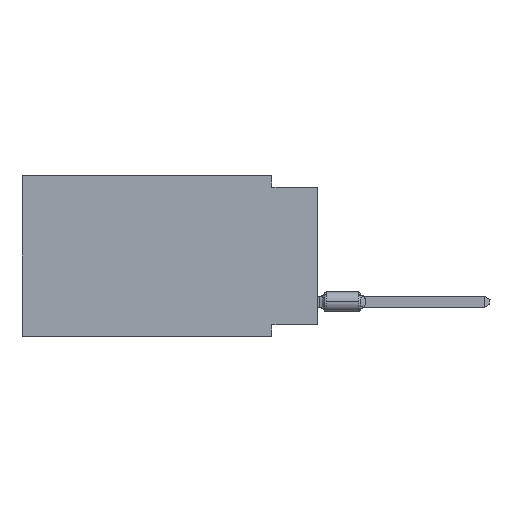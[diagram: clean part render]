
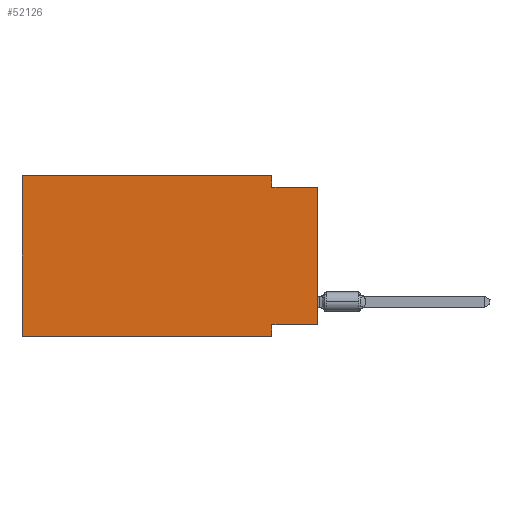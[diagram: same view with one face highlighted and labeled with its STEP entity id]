
A CAD part, left-side view. The second image highlights one B-rep face of the part: STEP entity #52126.
In plain terms, the highlighted planar face has unit normal (-1, 0, 0).
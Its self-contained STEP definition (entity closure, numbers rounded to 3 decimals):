
#1 = VECTOR ( 'NONE', #99394, 1000. ) ;
#1912 = VERTEX_POINT ( 'NONE', #21549 ) ;
#3960 = ORIENTED_EDGE ( 'NONE', *, *, #40717, .F. ) ;
#4182 = DIRECTION ( 'NONE',  ( 0., 0., -1. ) ) ;
#7124 = VERTEX_POINT ( 'NONE', #81972 ) ;
#7628 = ORIENTED_EDGE ( 'NONE', *, *, #89636, .F. ) ;
#10782 = DIRECTION ( 'NONE',  ( 0., 0., -1. ) ) ;
#10893 = LINE ( 'NONE', #11415, #1 ) ;
#11415 = CARTESIAN_POINT ( 'NONE',  ( 0., 0., -0.635 ) ) ;
#11553 = CARTESIAN_POINT ( 'NONE',  ( 0., 16.383, 0. ) ) ;
#11763 = CARTESIAN_POINT ( 'NONE',  ( 0., 16.383, 0. ) ) ;
#11833 = LINE ( 'NONE', #36059, #82247 ) ;
#12794 = VERTEX_POINT ( 'NONE', #13997 ) ;
#13997 = CARTESIAN_POINT ( 'NONE',  ( 0., 16.383, -8.89 ) ) ;
#14413 = VERTEX_POINT ( 'NONE', #46054 ) ;
#17647 = EDGE_CURVE ( 'NONE', #39506, #90280, #42423, .T. ) ;
#17708 = EDGE_CURVE ( 'NONE', #12794, #90280, #11833, .T. ) ;
#17879 = VECTOR ( 'NONE', #26842, 1000. ) ;
#18206 = ORIENTED_EDGE ( 'NONE', *, *, #17708, .T. ) ;
#19656 = FACE_OUTER_BOUND ( 'NONE', #53741, .T. ) ;
#19682 = CARTESIAN_POINT ( 'NONE',  ( 0., 16.383, 0. ) ) ;
#21549 = CARTESIAN_POINT ( 'NONE',  ( 0., 0., -0.635 ) ) ;
#24743 = VERTEX_POINT ( 'NONE', #36303 ) ;
#26842 = DIRECTION ( 'NONE',  ( 0., 0., 1. ) ) ;
#27424 = EDGE_CURVE ( 'NONE', #7124, #55537, #98212, .T. ) ;
#28751 = ORIENTED_EDGE ( 'NONE', *, *, #27424, .F. ) ;
#29482 = EDGE_CURVE ( 'NONE', #24743, #1912, #68447, .T. ) ;
#36059 = CARTESIAN_POINT ( 'NONE',  ( 0., 16.383, -8.89 ) ) ;
#36303 = CARTESIAN_POINT ( 'NONE',  ( 0., 0., -8.255 ) ) ;
#37333 = DIRECTION ( 'NONE',  ( 0., 0., 1. ) ) ;
#39506 = VERTEX_POINT ( 'NONE', #102109 ) ;
#40717 = EDGE_CURVE ( 'NONE', #12794, #7124, #44740, .T. ) ;
#42423 = LINE ( 'NONE', #82987, #55319 ) ;
#43921 = DIRECTION ( 'NONE',  ( 1., 0., 0. ) ) ;
#44740 = LINE ( 'NONE', #11553, #17879 ) ;
#46054 = CARTESIAN_POINT ( 'NONE',  ( 0., 2.54, -0.635 ) ) ;
#46403 = CARTESIAN_POINT ( 'NONE',  ( 0., 0., -8.255 ) ) ;
#49022 = VECTOR ( 'NONE', #68158, 1000. ) ;
#52126 = ADVANCED_FACE ( 'NONE', ( #19656 ), #83963, .F. ) ;
#52921 = DIRECTION ( 'NONE',  ( 0., -1., 0. ) ) ;
#53741 = EDGE_LOOP ( 'NONE', ( #103125, #98669, #7628, #28751, #3960, #18206, #103099, #67487 ) ) ;
#54201 = CARTESIAN_POINT ( 'NONE',  ( 0., 0., 0. ) ) ;
#54928 = VECTOR ( 'NONE', #4182, 1000. ) ;
#55319 = VECTOR ( 'NONE', #10782, 1000. ) ;
#55537 = VERTEX_POINT ( 'NONE', #89894 ) ;
#60238 = EDGE_CURVE ( 'NONE', #24743, #39506, #62213, .T. ) ;
#62213 = LINE ( 'NONE', #46403, #78360 ) ;
#62346 = AXIS2_PLACEMENT_3D ( 'NONE', #11763, #43921, #76046 ) ;
#65824 = CARTESIAN_POINT ( 'NONE',  ( 0., 2.54, -8.89 ) ) ;
#67487 = ORIENTED_EDGE ( 'NONE', *, *, #60238, .F. ) ;
#68158 = DIRECTION ( 'NONE',  ( 0., -1., 0. ) ) ;
#68447 = LINE ( 'NONE', #54201, #87966 ) ;
#69592 = DIRECTION ( 'NONE',  ( 0., 1., 0. ) ) ;
#72010 = EDGE_CURVE ( 'NONE', #14413, #1912, #10893, .T. ) ;
#76046 = DIRECTION ( 'NONE',  ( 0., 0., -1. ) ) ;
#76363 = CARTESIAN_POINT ( 'NONE',  ( 0., 2.54, 0. ) ) ;
#76884 = LINE ( 'NONE', #76363, #54928 ) ;
#78360 = VECTOR ( 'NONE', #69592, 1000. ) ;
#81972 = CARTESIAN_POINT ( 'NONE',  ( 0., 16.383, 0. ) ) ;
#82247 = VECTOR ( 'NONE', #52921, 1000. ) ;
#82987 = CARTESIAN_POINT ( 'NONE',  ( 0., 2.54, -8.89 ) ) ;
#83963 = PLANE ( 'NONE',  #62346 ) ;
#87966 = VECTOR ( 'NONE', #37333, 1000. ) ;
#89636 = EDGE_CURVE ( 'NONE', #55537, #14413, #76884, .T. ) ;
#89894 = CARTESIAN_POINT ( 'NONE',  ( 0., 2.54, 0. ) ) ;
#90280 = VERTEX_POINT ( 'NONE', #65824 ) ;
#98212 = LINE ( 'NONE', #19682, #49022 ) ;
#98669 = ORIENTED_EDGE ( 'NONE', *, *, #72010, .F. ) ;
#99394 = DIRECTION ( 'NONE',  ( 0., -1., 0. ) ) ;
#102109 = CARTESIAN_POINT ( 'NONE',  ( 0., 2.54, -8.255 ) ) ;
#103099 = ORIENTED_EDGE ( 'NONE', *, *, #17647, .F. ) ;
#103125 = ORIENTED_EDGE ( 'NONE', *, *, #29482, .T. ) ;
